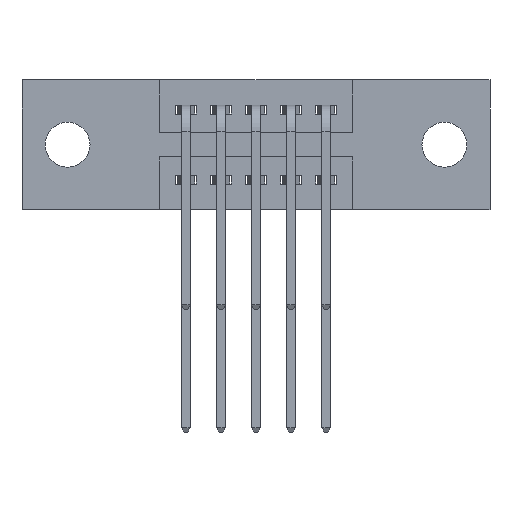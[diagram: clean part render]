
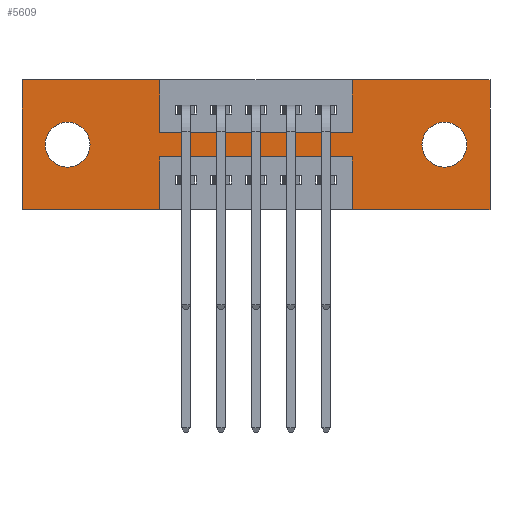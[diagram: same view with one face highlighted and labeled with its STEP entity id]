
A CAD part, front view. The second image highlights one B-rep face of the part: STEP entity #5609.
In plain terms, the highlighted planar face has unit normal (0, -1, 0).
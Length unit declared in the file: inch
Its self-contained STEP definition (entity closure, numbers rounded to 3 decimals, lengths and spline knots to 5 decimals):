
#61 = DIRECTION ( 'NONE',  ( 0., -1., 0. ) ) ;
#261 = DIRECTION ( 'NONE',  ( 0., 0., 1. ) ) ;
#309 = VERTEX_POINT ( 'NONE', #8410 ) ;
#352 = VERTEX_POINT ( 'NONE', #2858 ) ;
#380 = VECTOR ( 'NONE', #9858, 39.37008 ) ;
#456 = CARTESIAN_POINT ( 'NONE',  ( 0.13, 0., -0.121 ) ) ;
#572 = CARTESIAN_POINT ( 'NONE',  ( 0., 0., 0. ) ) ;
#685 = AXIS2_PLACEMENT_3D ( 'NONE', #5091, #4889, #7009 ) ;
#699 = LINE ( 'NONE', #9920, #380 ) ;
#701 = ORIENTED_EDGE ( 'NONE', *, *, #4701, .F. ) ;
#705 = VERTEX_POINT ( 'NONE', #1976 ) ;
#712 = CARTESIAN_POINT ( 'NONE',  ( 0., 0., 0. ) ) ;
#729 = CARTESIAN_POINT ( 'NONE',  ( 0.9425, 0., 0. ) ) ;
#862 = ORIENTED_EDGE ( 'NONE', *, *, #8775, .T. ) ;
#897 = LINE ( 'NONE', #7874, #5155 ) ;
#1047 = VERTEX_POINT ( 'NONE', #5053 ) ;
#1100 = ORIENTED_EDGE ( 'NONE', *, *, #8289, .F. ) ;
#1106 = ORIENTED_EDGE ( 'NONE', *, *, #5436, .F. ) ;
#1116 = ORIENTED_EDGE ( 'NONE', *, *, #5097, .T. ) ;
#1216 = CARTESIAN_POINT ( 'NONE',  ( 1.205, 0., -0.121 ) ) ;
#1317 = CIRCLE ( 'NONE', #9985, 0.064 ) ;
#1326 = CARTESIAN_POINT ( 'NONE',  ( 1.335, 0., -0.37 ) ) ;
#1389 = VERTEX_POINT ( 'NONE', #10038 ) ;
#1392 = LINE ( 'NONE', #6412, #5810 ) ;
#1493 = VECTOR ( 'NONE', #5797, 39.37008 ) ;
#1605 = VECTOR ( 'NONE', #9588, 39.37008 ) ;
#1661 = CARTESIAN_POINT ( 'NONE',  ( 0.13, 0., -0.185 ) ) ;
#1829 = CARTESIAN_POINT ( 'NONE',  ( 0.9425, 0., -0.37 ) ) ;
#1976 = CARTESIAN_POINT ( 'NONE',  ( 0.9425, 0., -0.15 ) ) ;
#2268 = CARTESIAN_POINT ( 'NONE',  ( 0.3925, 0., -0.22 ) ) ;
#2328 = ORIENTED_EDGE ( 'NONE', *, *, #3832, .F. ) ;
#2349 = EDGE_CURVE ( 'NONE', #5828, #6763, #699, .T. ) ;
#2559 = DIRECTION ( 'NONE',  ( 0., 0., 1. ) ) ;
#2586 = DIRECTION ( 'NONE',  ( 0., 1., 0. ) ) ;
#2609 = VERTEX_POINT ( 'NONE', #1326 ) ;
#2647 = LINE ( 'NONE', #4661, #8655 ) ;
#2667 = VECTOR ( 'NONE', #2963, 39.37008 ) ;
#2680 = VERTEX_POINT ( 'NONE', #456 ) ;
#2858 = CARTESIAN_POINT ( 'NONE',  ( 0.9425, 0., 0. ) ) ;
#2963 = DIRECTION ( 'NONE',  ( 1., 0., 0. ) ) ;
#3076 = VERTEX_POINT ( 'NONE', #6964 ) ;
#3248 = DIRECTION ( 'NONE',  ( 0., 0., -1. ) ) ;
#3295 = ORIENTED_EDGE ( 'NONE', *, *, #4304, .F. ) ;
#3564 = ORIENTED_EDGE ( 'NONE', *, *, #4624, .F. ) ;
#3824 = LINE ( 'NONE', #5010, #1493 ) ;
#3832 = EDGE_CURVE ( 'NONE', #9370, #3076, #5109, .T. ) ;
#3935 = VECTOR ( 'NONE', #5009, 39.37008 ) ;
#4044 = EDGE_LOOP ( 'NONE', ( #1116, #862 ) ) ;
#4265 = AXIS2_PLACEMENT_3D ( 'NONE', #7307, #2586, #8087 ) ;
#4304 = EDGE_CURVE ( 'NONE', #2609, #5550, #8425, .T. ) ;
#4567 = CIRCLE ( 'NONE', #9900, 0.064 ) ;
#4583 = EDGE_LOOP ( 'NONE', ( #5286, #3564, #1106, #3295, #701, #7260, #10379, #1100, #4965, #2328, #5645, #6446 ) ) ;
#4624 = EDGE_CURVE ( 'NONE', #1389, #5828, #1392, .T. ) ;
#4648 = DIRECTION ( 'NONE',  ( 0., 1., 0. ) ) ;
#4661 = CARTESIAN_POINT ( 'NONE',  ( 1.335, 0., 0. ) ) ;
#4701 = EDGE_CURVE ( 'NONE', #309, #2609, #2647, .T. ) ;
#4819 = ORIENTED_EDGE ( 'NONE', *, *, #9437, .T. ) ;
#4875 = VERTEX_POINT ( 'NONE', #10061 ) ;
#4889 = DIRECTION ( 'NONE',  ( 0., 1., 0. ) ) ;
#4965 = ORIENTED_EDGE ( 'NONE', *, *, #9898, .F. ) ;
#4981 = EDGE_LOOP ( 'NONE', ( #4819, #8863 ) ) ;
#5009 = DIRECTION ( 'NONE',  ( 1., 0., 0. ) ) ;
#5010 = CARTESIAN_POINT ( 'NONE',  ( 0., 0., 0. ) ) ;
#5053 = CARTESIAN_POINT ( 'NONE',  ( 1.205, 0., -0.249 ) ) ;
#5091 = CARTESIAN_POINT ( 'NONE',  ( 0.13, 0., -0.185 ) ) ;
#5097 = EDGE_CURVE ( 'NONE', #2680, #8011, #9146, .T. ) ;
#5109 = LINE ( 'NONE', #572, #2667 ) ;
#5155 = VECTOR ( 'NONE', #8650, 39.37008 ) ;
#5275 = PLANE ( 'NONE',  #6420 ) ;
#5286 = ORIENTED_EDGE ( 'NONE', *, *, #2349, .F. ) ;
#5436 = EDGE_CURVE ( 'NONE', #5550, #1389, #8042, .T. ) ;
#5550 = VERTEX_POINT ( 'NONE', #1829 ) ;
#5572 = EDGE_CURVE ( 'NONE', #705, #352, #8397, .T. ) ;
#5576 = DIRECTION ( 'NONE',  ( -1., 0., 0. ) ) ;
#5601 = CIRCLE ( 'NONE', #4265, 0.064 ) ;
#5609 = ADVANCED_FACE ( 'NONE', ( #9998, #5908, #7913 ), #5275, .T. ) ;
#5645 = ORIENTED_EDGE ( 'NONE', *, *, #6451, .F. ) ;
#5707 = CARTESIAN_POINT ( 'NONE',  ( 0., 0., 0. ) ) ;
#5797 = DIRECTION ( 'NONE',  ( 0., 0., 1. ) ) ;
#5810 = VECTOR ( 'NONE', #7124, 39.37008 ) ;
#5828 = VERTEX_POINT ( 'NONE', #2268 ) ;
#5841 = VECTOR ( 'NONE', #3248, 39.37008 ) ;
#5908 = FACE_BOUND ( 'NONE', #4044, .T. ) ;
#6042 = DIRECTION ( 'NONE',  ( 0., 0., -1. ) ) ;
#6200 = CARTESIAN_POINT ( 'NONE',  ( 0.13, 0., -0.249 ) ) ;
#6387 = VECTOR ( 'NONE', #261, 39.37008 ) ;
#6412 = CARTESIAN_POINT ( 'NONE',  ( 0.3925, 0., -0.22 ) ) ;
#6420 = AXIS2_PLACEMENT_3D ( 'NONE', #9873, #61, #6042 ) ;
#6446 = ORIENTED_EDGE ( 'NONE', *, *, #8183, .F. ) ;
#6451 = EDGE_CURVE ( 'NONE', #9974, #9370, #3824, .T. ) ;
#6497 = CARTESIAN_POINT ( 'NONE',  ( 0.3925, 0., -0.15 ) ) ;
#6653 = VECTOR ( 'NONE', #5576, 39.37008 ) ;
#6763 = VERTEX_POINT ( 'NONE', #9958 ) ;
#6964 = CARTESIAN_POINT ( 'NONE',  ( 0.3925, 0., 0. ) ) ;
#7009 = DIRECTION ( 'NONE',  ( 0., 0., 1. ) ) ;
#7099 = DIRECTION ( 'NONE',  ( 0., 0., -1. ) ) ;
#7124 = DIRECTION ( 'NONE',  ( -1., 0., 0. ) ) ;
#7260 = ORIENTED_EDGE ( 'NONE', *, *, #8301, .F. ) ;
#7289 = DIRECTION ( 'NONE',  ( 0., 1., 0. ) ) ;
#7307 = CARTESIAN_POINT ( 'NONE',  ( 1.205, 0., -0.185 ) ) ;
#7341 = EDGE_CURVE ( 'NONE', #1047, #9743, #4567, .T. ) ;
#7870 = CARTESIAN_POINT ( 'NONE',  ( 0.3925, 0., 0. ) ) ;
#7874 = CARTESIAN_POINT ( 'NONE',  ( 0., 0., -0.37 ) ) ;
#7913 = FACE_OUTER_BOUND ( 'NONE', #4583, .T. ) ;
#8009 = LINE ( 'NONE', #6497, #3935 ) ;
#8011 = VERTEX_POINT ( 'NONE', #6200 ) ;
#8042 = LINE ( 'NONE', #9135, #8269 ) ;
#8087 = DIRECTION ( 'NONE',  ( 0., 0., -1. ) ) ;
#8183 = EDGE_CURVE ( 'NONE', #6763, #9974, #897, .T. ) ;
#8269 = VECTOR ( 'NONE', #8890, 39.37008 ) ;
#8289 = EDGE_CURVE ( 'NONE', #4875, #705, #8009, .T. ) ;
#8301 = EDGE_CURVE ( 'NONE', #352, #309, #9826, .T. ) ;
#8397 = LINE ( 'NONE', #729, #6387 ) ;
#8410 = CARTESIAN_POINT ( 'NONE',  ( 1.335, 0., 0. ) ) ;
#8425 = LINE ( 'NONE', #9290, #6653 ) ;
#8650 = DIRECTION ( 'NONE',  ( -1., 0., 0. ) ) ;
#8655 = VECTOR ( 'NONE', #7099, 39.37008 ) ;
#8775 = EDGE_CURVE ( 'NONE', #8011, #2680, #1317, .T. ) ;
#8863 = ORIENTED_EDGE ( 'NONE', *, *, #7341, .T. ) ;
#8890 = DIRECTION ( 'NONE',  ( 0., 0., 1. ) ) ;
#9135 = CARTESIAN_POINT ( 'NONE',  ( 0.9425, 0., -0.37 ) ) ;
#9146 = CIRCLE ( 'NONE', #685, 0.064 ) ;
#9229 = CARTESIAN_POINT ( 'NONE',  ( 1.205, 0., -0.185 ) ) ;
#9290 = CARTESIAN_POINT ( 'NONE',  ( 0., 0., -0.37 ) ) ;
#9370 = VERTEX_POINT ( 'NONE', #5707 ) ;
#9437 = EDGE_CURVE ( 'NONE', #9743, #1047, #5601, .T. ) ;
#9588 = DIRECTION ( 'NONE',  ( 1., 0., 0. ) ) ;
#9676 = LINE ( 'NONE', #7870, #5841 ) ;
#9743 = VERTEX_POINT ( 'NONE', #1216 ) ;
#9826 = LINE ( 'NONE', #712, #1605 ) ;
#9858 = DIRECTION ( 'NONE',  ( 0., 0., -1. ) ) ;
#9873 = CARTESIAN_POINT ( 'NONE',  ( 0., 0., -0.37 ) ) ;
#9898 = EDGE_CURVE ( 'NONE', #3076, #4875, #9676, .T. ) ;
#9900 = AXIS2_PLACEMENT_3D ( 'NONE', #9229, #4648, #10018 ) ;
#9920 = CARTESIAN_POINT ( 'NONE',  ( 0.3925, 0., -0.37 ) ) ;
#9958 = CARTESIAN_POINT ( 'NONE',  ( 0.3925, 0., -0.37 ) ) ;
#9974 = VERTEX_POINT ( 'NONE', #10308 ) ;
#9985 = AXIS2_PLACEMENT_3D ( 'NONE', #1661, #7289, #2559 ) ;
#9998 = FACE_BOUND ( 'NONE', #4981, .T. ) ;
#10018 = DIRECTION ( 'NONE',  ( 0., 0., -1. ) ) ;
#10038 = CARTESIAN_POINT ( 'NONE',  ( 0.9425, 0., -0.22 ) ) ;
#10061 = CARTESIAN_POINT ( 'NONE',  ( 0.3925, 0., -0.15 ) ) ;
#10308 = CARTESIAN_POINT ( 'NONE',  ( 0., 0., -0.37 ) ) ;
#10379 = ORIENTED_EDGE ( 'NONE', *, *, #5572, .F. ) ;
